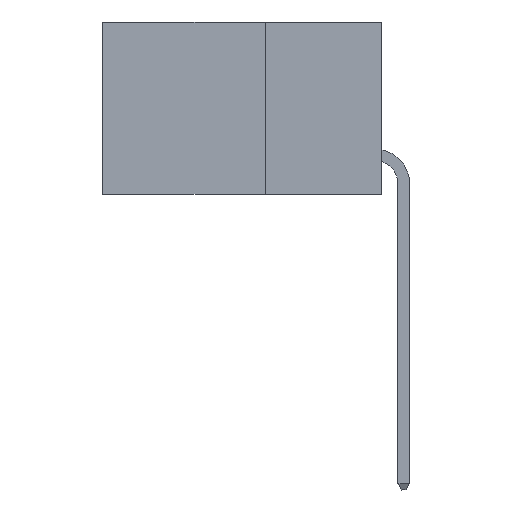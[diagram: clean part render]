
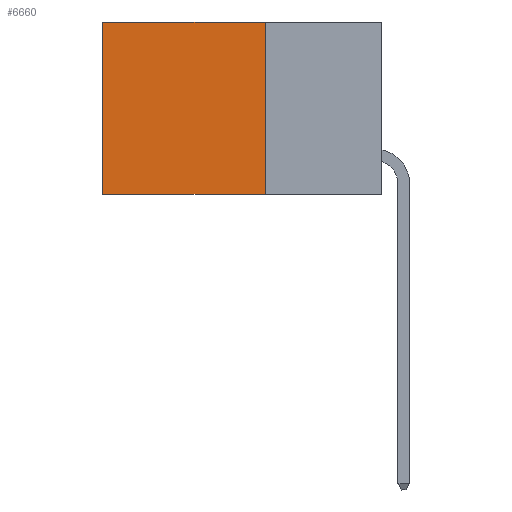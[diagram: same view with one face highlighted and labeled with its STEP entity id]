
A CAD part, left-side view. The second image highlights one B-rep face of the part: STEP entity #6660.
In plain terms, the highlighted planar face has unit normal (-1, 0, 0).
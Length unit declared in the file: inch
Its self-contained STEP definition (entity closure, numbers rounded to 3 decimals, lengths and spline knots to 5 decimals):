
#34 = EDGE_CURVE ( 'NONE', #602, #7554, #2582, .T. ) ;
#602 = VERTEX_POINT ( 'NONE', #17977 ) ;
#1362 = CARTESIAN_POINT ( 'NONE',  ( 0.2875, 0.25, -0.37 ) ) ;
#1609 = DIRECTION ( 'NONE',  ( 1., 0., 0. ) ) ;
#2088 = DIRECTION ( 'NONE',  ( 0., 1., 0. ) ) ;
#2582 = LINE ( 'NONE', #22868, #13863 ) ;
#3114 = LINE ( 'NONE', #25917, #8783 ) ;
#5766 = VECTOR ( 'NONE', #11230, 39.37008 ) ;
#6660 = ADVANCED_FACE ( 'NONE', ( #9029 ), #13655, .F. ) ;
#6771 = ORIENTED_EDGE ( 'NONE', *, *, #9923, .T. ) ;
#7312 = CARTESIAN_POINT ( 'NONE',  ( 0.2875, 0.25, 0. ) ) ;
#7524 = EDGE_CURVE ( 'NONE', #602, #11825, #28310, .T. ) ;
#7554 = VERTEX_POINT ( 'NONE', #12163 ) ;
#8159 = ORIENTED_EDGE ( 'NONE', *, *, #34, .T. ) ;
#8783 = VECTOR ( 'NONE', #2088, 39.37008 ) ;
#9029 = FACE_OUTER_BOUND ( 'NONE', #14757, .T. ) ;
#9749 = CARTESIAN_POINT ( 'NONE',  ( 0.2875, 0.6, -0.37 ) ) ;
#9923 = EDGE_CURVE ( 'NONE', #7554, #19649, #12193, .T. ) ;
#11230 = DIRECTION ( 'NONE',  ( 0., 0., -1. ) ) ;
#11724 = ORIENTED_EDGE ( 'NONE', *, *, #7524, .F. ) ;
#11825 = VERTEX_POINT ( 'NONE', #1362 ) ;
#12163 = CARTESIAN_POINT ( 'NONE',  ( 0.2875, 0.6, 0. ) ) ;
#12193 = LINE ( 'NONE', #20712, #5766 ) ;
#12887 = AXIS2_PLACEMENT_3D ( 'NONE', #30234, #1609, #18447 ) ;
#13655 = PLANE ( 'NONE',  #12887 ) ;
#13863 = VECTOR ( 'NONE', #22251, 39.37008 ) ;
#14757 = EDGE_LOOP ( 'NONE', ( #6771, #29437, #11724, #8159 ) ) ;
#16126 = EDGE_CURVE ( 'NONE', #11825, #19649, #3114, .T. ) ;
#17977 = CARTESIAN_POINT ( 'NONE',  ( 0.2875, 0.25, 0. ) ) ;
#18447 = DIRECTION ( 'NONE',  ( 0., 0., -1. ) ) ;
#19649 = VERTEX_POINT ( 'NONE', #9749 ) ;
#20712 = CARTESIAN_POINT ( 'NONE',  ( 0.2875, 0.6, 0. ) ) ;
#21616 = DIRECTION ( 'NONE',  ( 0., 0., -1. ) ) ;
#22033 = VECTOR ( 'NONE', #21616, 39.37008 ) ;
#22251 = DIRECTION ( 'NONE',  ( 0., 1., 0. ) ) ;
#22868 = CARTESIAN_POINT ( 'NONE',  ( 0.2875, 0.25, 0. ) ) ;
#25917 = CARTESIAN_POINT ( 'NONE',  ( 0.2875, 0.25, -0.37 ) ) ;
#28310 = LINE ( 'NONE', #7312, #22033 ) ;
#29437 = ORIENTED_EDGE ( 'NONE', *, *, #16126, .F. ) ;
#30234 = CARTESIAN_POINT ( 'NONE',  ( 0.2875, 0.25, 0. ) ) ;
